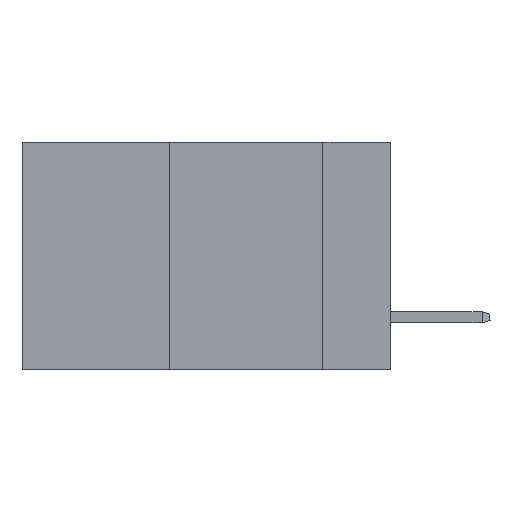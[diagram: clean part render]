
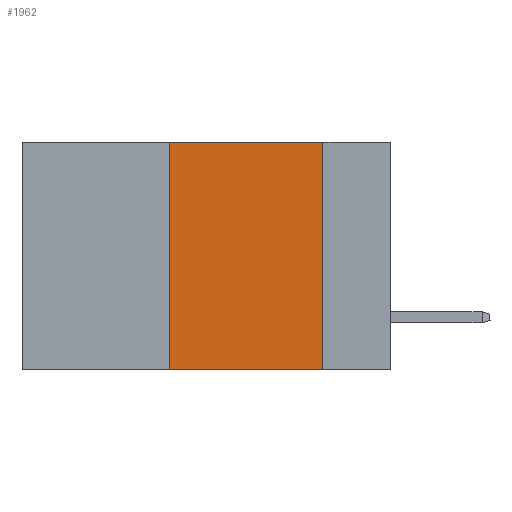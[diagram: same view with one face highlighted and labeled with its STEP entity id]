
A CAD part, left-side view. The second image highlights one B-rep face of the part: STEP entity #1962.
In plain terms, the highlighted planar face has unit normal (-1, 0, 0).
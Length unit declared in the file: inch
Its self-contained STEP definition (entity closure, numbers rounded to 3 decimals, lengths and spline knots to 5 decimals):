
#238 = DIRECTION ( 'NONE',  ( 0., -1., 0. ) ) ;
#274 = CARTESIAN_POINT ( 'NONE',  ( 0., 0.36, 0. ) ) ;
#705 = VERTEX_POINT ( 'NONE', #2488 ) ;
#1962 = ADVANCED_FACE ( 'NONE', ( #14061 ), #10663, .F. ) ;
#2488 = CARTESIAN_POINT ( 'NONE',  ( 0., 0.36, -0.37 ) ) ;
#2783 = LINE ( 'NONE', #17568, #13171 ) ;
#2819 = LINE ( 'NONE', #15120, #15547 ) ;
#2866 = VECTOR ( 'NONE', #4633, 39.37008 ) ;
#3022 = ORIENTED_EDGE ( 'NONE', *, *, #12237, .F. ) ;
#3532 = CARTESIAN_POINT ( 'NONE',  ( 0., 0.11, 0. ) ) ;
#3888 = LINE ( 'NONE', #5416, #5370 ) ;
#4237 = AXIS2_PLACEMENT_3D ( 'NONE', #9229, #15873, #6493 ) ;
#4633 = DIRECTION ( 'NONE',  ( 0., 0., -1. ) ) ;
#5258 = ORIENTED_EDGE ( 'NONE', *, *, #10680, .F. ) ;
#5370 = VECTOR ( 'NONE', #238, 39.37008 ) ;
#5416 = CARTESIAN_POINT ( 'NONE',  ( 0., 0.6, -0.37 ) ) ;
#5635 = DIRECTION ( 'NONE',  ( 0., -1., 0. ) ) ;
#5811 = EDGE_LOOP ( 'NONE', ( #9522, #5258, #3022, #16216 ) ) ;
#6493 = DIRECTION ( 'NONE',  ( 0., 0., -1. ) ) ;
#8400 = VERTEX_POINT ( 'NONE', #16729 ) ;
#9229 = CARTESIAN_POINT ( 'NONE',  ( 0., 0.6, 0. ) ) ;
#9390 = EDGE_CURVE ( 'NONE', #14978, #8400, #16033, .T. ) ;
#9522 = ORIENTED_EDGE ( 'NONE', *, *, #9390, .F. ) ;
#10598 = EDGE_CURVE ( 'NONE', #705, #8400, #3888, .T. ) ;
#10663 = PLANE ( 'NONE',  #4237 ) ;
#10680 = EDGE_CURVE ( 'NONE', #17181, #14978, #2819, .T. ) ;
#12237 = EDGE_CURVE ( 'NONE', #705, #17181, #2783, .T. ) ;
#13171 = VECTOR ( 'NONE', #17506, 39.37008 ) ;
#14061 = FACE_OUTER_BOUND ( 'NONE', #5811, .T. ) ;
#14104 = CARTESIAN_POINT ( 'NONE',  ( 0., 0.11, 0. ) ) ;
#14978 = VERTEX_POINT ( 'NONE', #14104 ) ;
#15120 = CARTESIAN_POINT ( 'NONE',  ( 0., 0.6, 0. ) ) ;
#15547 = VECTOR ( 'NONE', #5635, 39.37008 ) ;
#15873 = DIRECTION ( 'NONE',  ( 1., 0., 0. ) ) ;
#16033 = LINE ( 'NONE', #3532, #2866 ) ;
#16216 = ORIENTED_EDGE ( 'NONE', *, *, #10598, .T. ) ;
#16729 = CARTESIAN_POINT ( 'NONE',  ( 0., 0.11, -0.37 ) ) ;
#17181 = VERTEX_POINT ( 'NONE', #274 ) ;
#17506 = DIRECTION ( 'NONE',  ( 0., 0., 1. ) ) ;
#17568 = CARTESIAN_POINT ( 'NONE',  ( 0., 0.36, 0. ) ) ;
